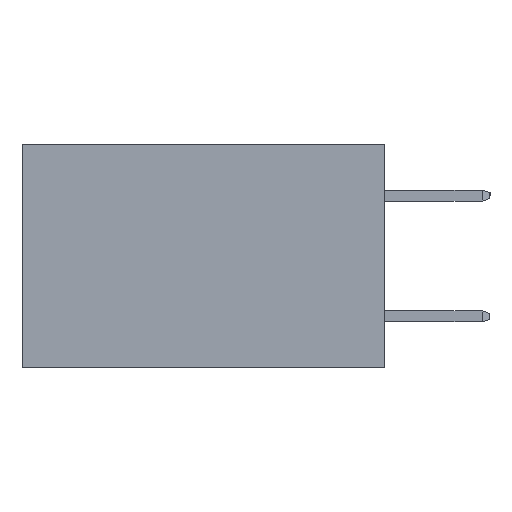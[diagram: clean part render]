
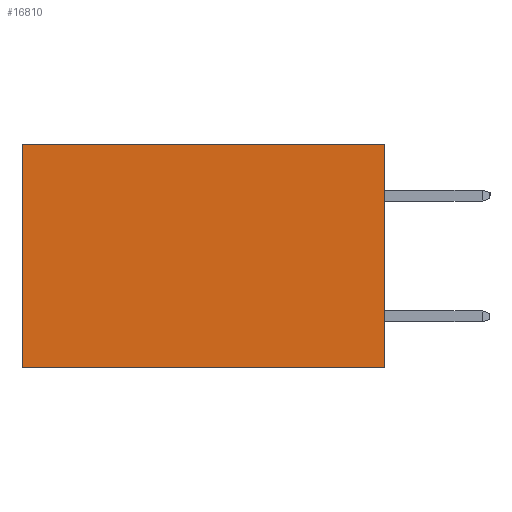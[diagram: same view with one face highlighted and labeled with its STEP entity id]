
A CAD part, left-side view. The second image highlights one B-rep face of the part: STEP entity #16810.
In plain terms, the highlighted planar face has unit normal (-1, 0, 0).
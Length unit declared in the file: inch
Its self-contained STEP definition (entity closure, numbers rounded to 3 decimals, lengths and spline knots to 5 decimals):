
#70 = ORIENTED_EDGE ( 'NONE', *, *, #16776, .F. ) ;
#83 = VERTEX_POINT ( 'NONE', #6785 ) ;
#802 = CARTESIAN_POINT ( 'NONE',  ( 0.2615, 0., -0.37 ) ) ;
#995 = FACE_OUTER_BOUND ( 'NONE', #1207, .T. ) ;
#1042 = EDGE_CURVE ( 'NONE', #14294, #9374, #15964, .T. ) ;
#1207 = EDGE_LOOP ( 'NONE', ( #15459, #70, #4476, #3232 ) ) ;
#1707 = AXIS2_PLACEMENT_3D ( 'NONE', #802, #8269, #8555 ) ;
#1749 = CARTESIAN_POINT ( 'NONE',  ( 0.2615, 0., -0.37 ) ) ;
#1983 = VECTOR ( 'NONE', #2265, 39.37008 ) ;
#2265 = DIRECTION ( 'NONE',  ( 0., 0., -1. ) ) ;
#3055 = CARTESIAN_POINT ( 'NONE',  ( 0.2615, 0.6, 0. ) ) ;
#3232 = ORIENTED_EDGE ( 'NONE', *, *, #1042, .T. ) ;
#3442 = DIRECTION ( 'NONE',  ( 0., 1., 0. ) ) ;
#3740 = VERTEX_POINT ( 'NONE', #1749 ) ;
#4476 = ORIENTED_EDGE ( 'NONE', *, *, #15886, .F. ) ;
#5995 = VECTOR ( 'NONE', #8806, 39.37008 ) ;
#6785 = CARTESIAN_POINT ( 'NONE',  ( 0.2615, 0.6, -0.37 ) ) ;
#7039 = LINE ( 'NONE', #17105, #9442 ) ;
#7132 = DIRECTION ( 'NONE',  ( 0., 0., -1. ) ) ;
#7452 = VECTOR ( 'NONE', #3442, 39.37008 ) ;
#8184 = CARTESIAN_POINT ( 'NONE',  ( 0.2615, 0., -0.37 ) ) ;
#8269 = DIRECTION ( 'NONE',  ( 1., 0., 0. ) ) ;
#8555 = DIRECTION ( 'NONE',  ( 0., 0., -1. ) ) ;
#8806 = DIRECTION ( 'NONE',  ( 0., 1., 0. ) ) ;
#9084 = CARTESIAN_POINT ( 'NONE',  ( 0.2615, 0., 0. ) ) ;
#9374 = VERTEX_POINT ( 'NONE', #3055 ) ;
#9425 = LINE ( 'NONE', #15188, #1983 ) ;
#9442 = VECTOR ( 'NONE', #7132, 39.37008 ) ;
#10817 = LINE ( 'NONE', #8184, #7452 ) ;
#12036 = PLANE ( 'NONE',  #1707 ) ;
#13641 = EDGE_CURVE ( 'NONE', #9374, #83, #7039, .T. ) ;
#14294 = VERTEX_POINT ( 'NONE', #14824 ) ;
#14824 = CARTESIAN_POINT ( 'NONE',  ( 0.2615, 0., 0. ) ) ;
#15188 = CARTESIAN_POINT ( 'NONE',  ( 0.2615, 0., -0.37 ) ) ;
#15459 = ORIENTED_EDGE ( 'NONE', *, *, #13641, .T. ) ;
#15886 = EDGE_CURVE ( 'NONE', #14294, #3740, #9425, .T. ) ;
#15964 = LINE ( 'NONE', #9084, #5995 ) ;
#16776 = EDGE_CURVE ( 'NONE', #3740, #83, #10817, .T. ) ;
#16810 = ADVANCED_FACE ( 'NONE', ( #995 ), #12036, .F. ) ;
#17105 = CARTESIAN_POINT ( 'NONE',  ( 0.2615, 0.6, -0.37 ) ) ;
